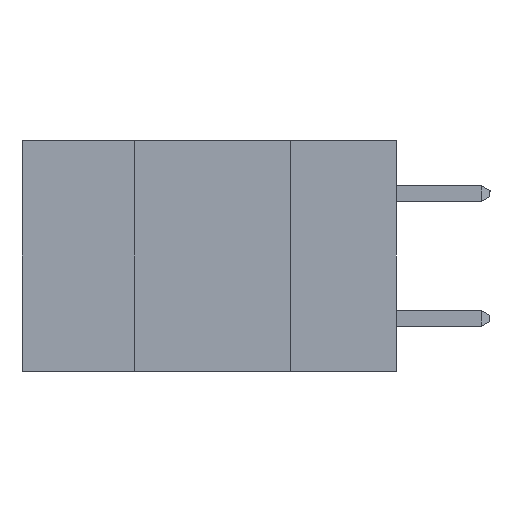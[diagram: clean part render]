
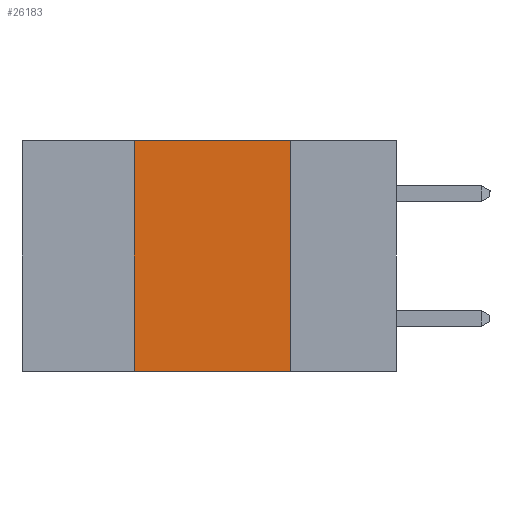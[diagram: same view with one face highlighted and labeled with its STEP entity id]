
A CAD part, left-side view. The second image highlights one B-rep face of the part: STEP entity #26183.
In plain terms, the highlighted planar face has unit normal (-1, 0, 0).
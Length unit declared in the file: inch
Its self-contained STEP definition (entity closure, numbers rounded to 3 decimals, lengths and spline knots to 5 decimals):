
#16 = LINE ( 'NONE', #14567, #18151 ) ;
#1041 = CARTESIAN_POINT ( 'NONE',  ( 0., 0.17, -0.37 ) ) ;
#1285 = ORIENTED_EDGE ( 'NONE', *, *, #3378, .F. ) ;
#2023 = CARTESIAN_POINT ( 'NONE',  ( 0., 0.42, -0.37 ) ) ;
#2678 = EDGE_CURVE ( 'NONE', #25434, #11164, #22860, .T. ) ;
#2699 = CARTESIAN_POINT ( 'NONE',  ( 0., 0.6, 0. ) ) ;
#3235 = VECTOR ( 'NONE', #20196, 39.37008 ) ;
#3378 = EDGE_CURVE ( 'NONE', #20561, #11164, #11936, .T. ) ;
#4117 = DIRECTION ( 'NONE',  ( 0., -1., 0. ) ) ;
#5314 = VECTOR ( 'NONE', #10324, 39.37008 ) ;
#6404 = CARTESIAN_POINT ( 'NONE',  ( 0., 0.42, 0. ) ) ;
#6667 = FACE_OUTER_BOUND ( 'NONE', #24633, .T. ) ;
#6804 = DIRECTION ( 'NONE',  ( 1., 0., 0. ) ) ;
#7168 = CARTESIAN_POINT ( 'NONE',  ( 0., 0.42, -0.37 ) ) ;
#9914 = ORIENTED_EDGE ( 'NONE', *, *, #2678, .T. ) ;
#10324 = DIRECTION ( 'NONE',  ( 0., 0., 1. ) ) ;
#10474 = DIRECTION ( 'NONE',  ( 0., 0., -1. ) ) ;
#11164 = VERTEX_POINT ( 'NONE', #1041 ) ;
#11661 = CARTESIAN_POINT ( 'NONE',  ( 0., 0.17, -0.37 ) ) ;
#11936 = LINE ( 'NONE', #11661, #3235 ) ;
#12423 = DIRECTION ( 'NONE',  ( 0., -1., 0. ) ) ;
#12773 = VECTOR ( 'NONE', #12423, 39.37008 ) ;
#13012 = ORIENTED_EDGE ( 'NONE', *, *, #13881, .F. ) ;
#13566 = AXIS2_PLACEMENT_3D ( 'NONE', #2699, #6804, #10474 ) ;
#13881 = EDGE_CURVE ( 'NONE', #25434, #26280, #14651, .T. ) ;
#13964 = ORIENTED_EDGE ( 'NONE', *, *, #18908, .F. ) ;
#14567 = CARTESIAN_POINT ( 'NONE',  ( 0., 0.6, 0. ) ) ;
#14651 = LINE ( 'NONE', #2023, #5314 ) ;
#16210 = CARTESIAN_POINT ( 'NONE',  ( 0., 0.6, -0.37 ) ) ;
#17249 = PLANE ( 'NONE',  #13566 ) ;
#18151 = VECTOR ( 'NONE', #4117, 39.37008 ) ;
#18908 = EDGE_CURVE ( 'NONE', #26280, #20561, #16, .T. ) ;
#19304 = CARTESIAN_POINT ( 'NONE',  ( 0., 0.17, 0. ) ) ;
#20196 = DIRECTION ( 'NONE',  ( 0., 0., -1. ) ) ;
#20561 = VERTEX_POINT ( 'NONE', #19304 ) ;
#22860 = LINE ( 'NONE', #16210, #12773 ) ;
#24633 = EDGE_LOOP ( 'NONE', ( #1285, #13964, #13012, #9914 ) ) ;
#25434 = VERTEX_POINT ( 'NONE', #7168 ) ;
#26183 = ADVANCED_FACE ( 'NONE', ( #6667 ), #17249, .F. ) ;
#26280 = VERTEX_POINT ( 'NONE', #6404 ) ;
